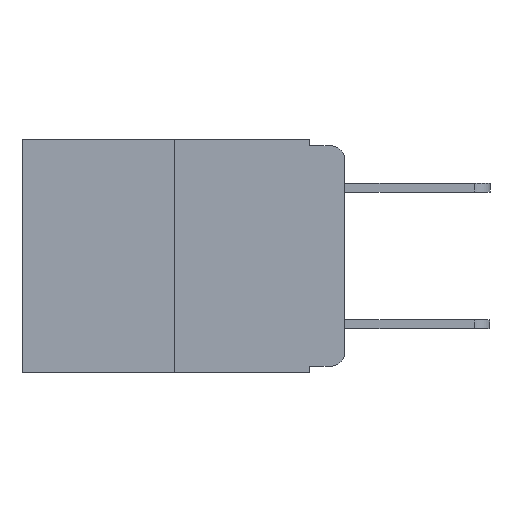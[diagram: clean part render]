
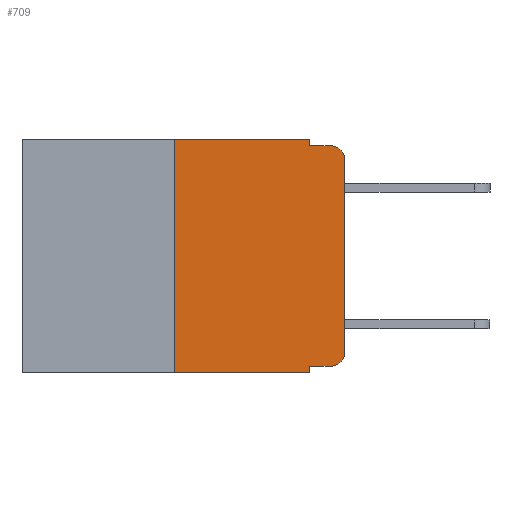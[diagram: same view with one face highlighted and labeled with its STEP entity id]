
A CAD part, left-side view. The second image highlights one B-rep face of the part: STEP entity #709.
In plain terms, the highlighted planar face has unit normal (-1, 0, 0).
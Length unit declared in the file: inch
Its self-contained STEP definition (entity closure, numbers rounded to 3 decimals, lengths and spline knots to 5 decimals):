
#128 = EDGE_CURVE ( 'NONE', #3701, #12467, #14587, .T. ) ;
#263 = EDGE_CURVE ( 'NONE', #9935, #15710, #4551, .T. ) ;
#490 = DIRECTION ( 'NONE',  ( 0., -1., 0. ) ) ;
#709 = ADVANCED_FACE ( 'NONE', ( #11918 ), #2939, .F. ) ;
#752 = CARTESIAN_POINT ( 'NONE',  ( 0., 0.02, -0.313 ) ) ;
#873 = EDGE_CURVE ( 'NONE', #3032, #15710, #15361, .T. ) ;
#889 = DIRECTION ( 'NONE',  ( -1., 0., 0. ) ) ;
#918 = EDGE_CURVE ( 'NONE', #15192, #2441, #18788, .T. ) ;
#1313 = DIRECTION ( 'NONE',  ( 0., 0., -1. ) ) ;
#1363 = DIRECTION ( 'NONE',  ( 0., -1., 0. ) ) ;
#1642 = CARTESIAN_POINT ( 'NONE',  ( 0., 0., -0.03 ) ) ;
#1901 = DIRECTION ( 'NONE',  ( 0., 0., 1. ) ) ;
#2246 = ORIENTED_EDGE ( 'NONE', *, *, #11865, .F. ) ;
#2360 = CARTESIAN_POINT ( 'NONE',  ( 0., 0.473, 0. ) ) ;
#2441 = VERTEX_POINT ( 'NONE', #8476 ) ;
#2518 = VECTOR ( 'NONE', #15202, 39.37008 ) ;
#2939 = PLANE ( 'NONE',  #14705 ) ;
#3032 = VERTEX_POINT ( 'NONE', #8043 ) ;
#3109 = EDGE_CURVE ( 'NONE', #9935, #15192, #10121, .T. ) ;
#3487 = CARTESIAN_POINT ( 'NONE',  ( 0., 0., 0. ) ) ;
#3558 = VECTOR ( 'NONE', #4494, 39.37008 ) ;
#3622 = CARTESIAN_POINT ( 'NONE',  ( 0., 0.25, 0. ) ) ;
#3701 = VERTEX_POINT ( 'NONE', #13607 ) ;
#4481 = VERTEX_POINT ( 'NONE', #11330 ) ;
#4494 = DIRECTION ( 'NONE',  ( 0., 0., -1. ) ) ;
#4551 = LINE ( 'NONE', #12886, #3558 ) ;
#5026 = VECTOR ( 'NONE', #11668, 39.37008 ) ;
#5684 = LINE ( 'NONE', #3487, #2518 ) ;
#5772 = CARTESIAN_POINT ( 'NONE',  ( 0., 0.473, -0.343 ) ) ;
#6214 = VECTOR ( 'NONE', #490, 39.37008 ) ;
#6323 = VECTOR ( 'NONE', #1901, 39.37008 ) ;
#6483 = DIRECTION ( 'NONE',  ( 0., 0., -1. ) ) ;
#6502 = DIRECTION ( 'NONE',  ( 1., 0., 0. ) ) ;
#7279 = VERTEX_POINT ( 'NONE', #1642 ) ;
#7362 = DIRECTION ( 'NONE',  ( 0., -1., 0. ) ) ;
#7631 = CARTESIAN_POINT ( 'NONE',  ( 0., 0.051, -0.343 ) ) ;
#8043 = CARTESIAN_POINT ( 'NONE',  ( 0., 0.25, -0.343 ) ) ;
#8476 = CARTESIAN_POINT ( 'NONE',  ( 0., 0., -0.313 ) ) ;
#8481 = EDGE_LOOP ( 'NONE', ( #11644, #11721, #13196, #11938, #12013, #2246, #12208, #12108, #12293, #12262 ) ) ;
#8503 = EDGE_CURVE ( 'NONE', #12467, #10957, #16388, .T. ) ;
#8752 = DIRECTION ( 'NONE',  ( -1., 0., 0. ) ) ;
#8803 = VECTOR ( 'NONE', #1363, 39.37008 ) ;
#9176 = CIRCLE ( 'NONE', #12236, 0.02 ) ;
#9321 = CARTESIAN_POINT ( 'NONE',  ( 0., 0.051, -0.01 ) ) ;
#9349 = LINE ( 'NONE', #11605, #5026 ) ;
#9453 = AXIS2_PLACEMENT_3D ( 'NONE', #752, #889, #1313 ) ;
#9935 = VERTEX_POINT ( 'NONE', #18908 ) ;
#10121 = LINE ( 'NONE', #16145, #6214 ) ;
#10232 = LINE ( 'NONE', #3622, #6323 ) ;
#10735 = VECTOR ( 'NONE', #12437, 39.37008 ) ;
#10957 = VERTEX_POINT ( 'NONE', #16367 ) ;
#11253 = EDGE_CURVE ( 'NONE', #2441, #7279, #5684, .T. ) ;
#11330 = CARTESIAN_POINT ( 'NONE',  ( 0., 0.25, 0. ) ) ;
#11600 = VECTOR ( 'NONE', #7362, 39.37008 ) ;
#11605 = CARTESIAN_POINT ( 'NONE',  ( 0., 0.473, 0. ) ) ;
#11644 = ORIENTED_EDGE ( 'NONE', *, *, #11253, .T. ) ;
#11668 = DIRECTION ( 'NONE',  ( 0., -1., 0. ) ) ;
#11721 = ORIENTED_EDGE ( 'NONE', *, *, #16274, .T. ) ;
#11865 = EDGE_CURVE ( 'NONE', #3032, #4481, #10232, .T. ) ;
#11918 = FACE_OUTER_BOUND ( 'NONE', #8481, .T. ) ;
#11938 = ORIENTED_EDGE ( 'NONE', *, *, #128, .F. ) ;
#12013 = ORIENTED_EDGE ( 'NONE', *, *, #18260, .F. ) ;
#12108 = ORIENTED_EDGE ( 'NONE', *, *, #263, .F. ) ;
#12208 = ORIENTED_EDGE ( 'NONE', *, *, #873, .T. ) ;
#12236 = AXIS2_PLACEMENT_3D ( 'NONE', #17211, #8752, #18506 ) ;
#12262 = ORIENTED_EDGE ( 'NONE', *, *, #918, .T. ) ;
#12293 = ORIENTED_EDGE ( 'NONE', *, *, #3109, .T. ) ;
#12437 = DIRECTION ( 'NONE',  ( 0., 0., -1. ) ) ;
#12467 = VERTEX_POINT ( 'NONE', #9321 ) ;
#12636 = CARTESIAN_POINT ( 'NONE',  ( 0., 0.051, 0. ) ) ;
#12886 = CARTESIAN_POINT ( 'NONE',  ( 0., 0.051, 0. ) ) ;
#13196 = ORIENTED_EDGE ( 'NONE', *, *, #8503, .F. ) ;
#13607 = CARTESIAN_POINT ( 'NONE',  ( 0., 0.051, 0. ) ) ;
#14051 = CARTESIAN_POINT ( 'NONE',  ( 0., 0.02, -0.333 ) ) ;
#14587 = LINE ( 'NONE', #12636, #10735 ) ;
#14705 = AXIS2_PLACEMENT_3D ( 'NONE', #2360, #6502, #6483 ) ;
#15192 = VERTEX_POINT ( 'NONE', #14051 ) ;
#15202 = DIRECTION ( 'NONE',  ( 0., 0., 1. ) ) ;
#15361 = LINE ( 'NONE', #5772, #11600 ) ;
#15710 = VERTEX_POINT ( 'NONE', #7631 ) ;
#16145 = CARTESIAN_POINT ( 'NONE',  ( 0., 0.051, -0.333 ) ) ;
#16274 = EDGE_CURVE ( 'NONE', #7279, #10957, #9176, .T. ) ;
#16367 = CARTESIAN_POINT ( 'NONE',  ( 0., 0.02, -0.01 ) ) ;
#16388 = LINE ( 'NONE', #18684, #8803 ) ;
#17211 = CARTESIAN_POINT ( 'NONE',  ( 0., 0.02, -0.03 ) ) ;
#18260 = EDGE_CURVE ( 'NONE', #4481, #3701, #9349, .T. ) ;
#18506 = DIRECTION ( 'NONE',  ( 0., 0., -1. ) ) ;
#18684 = CARTESIAN_POINT ( 'NONE',  ( 0., 0.051, -0.01 ) ) ;
#18788 = CIRCLE ( 'NONE', #9453, 0.02 ) ;
#18908 = CARTESIAN_POINT ( 'NONE',  ( 0., 0.051, -0.333 ) ) ;
